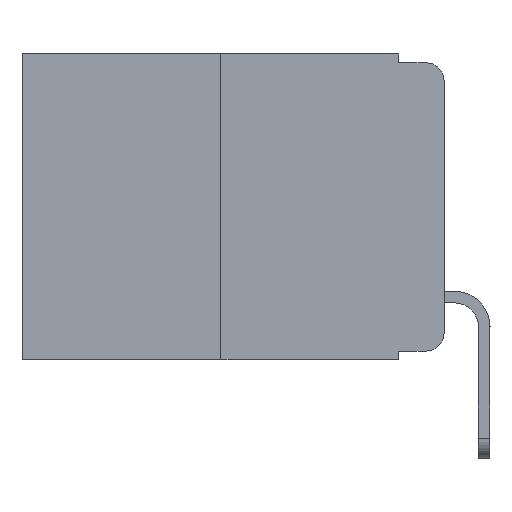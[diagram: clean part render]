
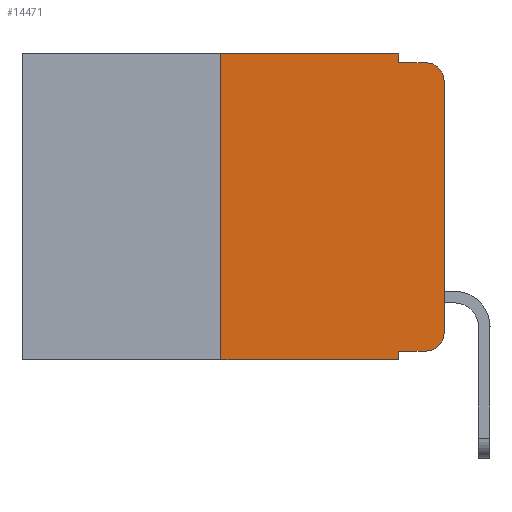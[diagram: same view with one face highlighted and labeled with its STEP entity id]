
A CAD part, left-side view. The second image highlights one B-rep face of the part: STEP entity #14471.
In plain terms, the highlighted planar face has unit normal (-1, 0, 0).
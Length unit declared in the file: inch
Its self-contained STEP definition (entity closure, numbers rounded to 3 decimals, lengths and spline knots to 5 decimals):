
#136 = EDGE_CURVE ( 'NONE', #6566, #16333, #18032, .T. ) ;
#454 = CIRCLE ( 'NONE', #20609, 0.02 ) ;
#620 = VECTOR ( 'NONE', #8441, 39.37008 ) ;
#773 = DIRECTION ( 'NONE',  ( 0., 0., -1. ) ) ;
#874 = CARTESIAN_POINT ( 'NONE',  ( 0., 0., 0. ) ) ;
#1082 = CARTESIAN_POINT ( 'NONE',  ( 0., 0.051, -0.333 ) ) ;
#1145 = ORIENTED_EDGE ( 'NONE', *, *, #17601, .F. ) ;
#1673 = AXIS2_PLACEMENT_3D ( 'NONE', #13457, #3919, #19971 ) ;
#1812 = CARTESIAN_POINT ( 'NONE',  ( 0., 0.051, -0.01 ) ) ;
#2244 = CARTESIAN_POINT ( 'NONE',  ( 0., 0.02, -0.01 ) ) ;
#2411 = DIRECTION ( 'NONE',  ( 0., -1., 0. ) ) ;
#2472 = LINE ( 'NONE', #874, #5906 ) ;
#2485 = VERTEX_POINT ( 'NONE', #20953 ) ;
#2672 = ORIENTED_EDGE ( 'NONE', *, *, #7482, .F. ) ;
#2871 = LINE ( 'NONE', #18800, #11596 ) ;
#3030 = VECTOR ( 'NONE', #3941, 39.37008 ) ;
#3312 = CARTESIAN_POINT ( 'NONE',  ( 0., 0.051, -0.01 ) ) ;
#3919 = DIRECTION ( 'NONE',  ( -1., 0., 0. ) ) ;
#3941 = DIRECTION ( 'NONE',  ( 0., -1., 0. ) ) ;
#4145 = DIRECTION ( 'NONE',  ( 0., 0., -1. ) ) ;
#4164 = LINE ( 'NONE', #1082, #3030 ) ;
#4324 = FACE_OUTER_BOUND ( 'NONE', #7030, .T. ) ;
#4434 = CARTESIAN_POINT ( 'NONE',  ( 0., 0.473, 0. ) ) ;
#4699 = CARTESIAN_POINT ( 'NONE',  ( 0., 0.25, -0.343 ) ) ;
#4918 = ORIENTED_EDGE ( 'NONE', *, *, #19283, .T. ) ;
#5364 = EDGE_CURVE ( 'NONE', #15579, #19111, #13482, .T. ) ;
#5436 = CARTESIAN_POINT ( 'NONE',  ( 0., 0.02, -0.03 ) ) ;
#5811 = ORIENTED_EDGE ( 'NONE', *, *, #136, .F. ) ;
#5906 = VECTOR ( 'NONE', #8766, 39.37008 ) ;
#5965 = EDGE_CURVE ( 'NONE', #15011, #9621, #8146, .T. ) ;
#6119 = CARTESIAN_POINT ( 'NONE',  ( 0., 0., -0.313 ) ) ;
#6271 = DIRECTION ( 'NONE',  ( 0., 0., 1. ) ) ;
#6566 = VERTEX_POINT ( 'NONE', #4699 ) ;
#6877 = LINE ( 'NONE', #18754, #10535 ) ;
#7030 = EDGE_LOOP ( 'NONE', ( #17421, #7716, #11924, #2672, #1145, #5811, #17931, #9835, #4918, #8713 ) ) ;
#7343 = CARTESIAN_POINT ( 'NONE',  ( 0., 0.473, -0.343 ) ) ;
#7482 = EDGE_CURVE ( 'NONE', #15963, #15579, #15278, .T. ) ;
#7559 = DIRECTION ( 'NONE',  ( 0., 0., -1. ) ) ;
#7569 = VERTEX_POINT ( 'NONE', #14309 ) ;
#7595 = EDGE_CURVE ( 'NONE', #6566, #8655, #15499, .T. ) ;
#7716 = ORIENTED_EDGE ( 'NONE', *, *, #12197, .T. ) ;
#7853 = PLANE ( 'NONE',  #12795 ) ;
#8031 = VECTOR ( 'NONE', #6271, 39.37008 ) ;
#8146 = CIRCLE ( 'NONE', #1673, 0.02 ) ;
#8441 = DIRECTION ( 'NONE',  ( 0., -1., 0. ) ) ;
#8655 = VERTEX_POINT ( 'NONE', #10343 ) ;
#8713 = ORIENTED_EDGE ( 'NONE', *, *, #5965, .T. ) ;
#8764 = EDGE_CURVE ( 'NONE', #7569, #8655, #2871, .T. ) ;
#8766 = DIRECTION ( 'NONE',  ( 0., 0., 1. ) ) ;
#9621 = VERTEX_POINT ( 'NONE', #6119 ) ;
#9835 = ORIENTED_EDGE ( 'NONE', *, *, #8764, .F. ) ;
#9902 = CARTESIAN_POINT ( 'NONE',  ( 0., 0.25, 0. ) ) ;
#10343 = CARTESIAN_POINT ( 'NONE',  ( 0., 0.051, -0.343 ) ) ;
#10535 = VECTOR ( 'NONE', #2411, 39.37008 ) ;
#10690 = DIRECTION ( 'NONE',  ( -1., 0., 0. ) ) ;
#10965 = DIRECTION ( 'NONE',  ( 0., 0., -1. ) ) ;
#11591 = CARTESIAN_POINT ( 'NONE',  ( 0., 0.25, 0. ) ) ;
#11596 = VECTOR ( 'NONE', #7559, 39.37008 ) ;
#11614 = VECTOR ( 'NONE', #4145, 39.37008 ) ;
#11924 = ORIENTED_EDGE ( 'NONE', *, *, #5364, .F. ) ;
#12197 = EDGE_CURVE ( 'NONE', #2485, #19111, #454, .T. ) ;
#12246 = EDGE_CURVE ( 'NONE', #9621, #2485, #2472, .T. ) ;
#12795 = AXIS2_PLACEMENT_3D ( 'NONE', #4434, #12798, #10965 ) ;
#12798 = DIRECTION ( 'NONE',  ( 1., 0., 0. ) ) ;
#13457 = CARTESIAN_POINT ( 'NONE',  ( 0., 0.02, -0.313 ) ) ;
#13482 = LINE ( 'NONE', #3312, #620 ) ;
#14001 = DIRECTION ( 'NONE',  ( 0., -1., 0. ) ) ;
#14309 = CARTESIAN_POINT ( 'NONE',  ( 0., 0.051, -0.333 ) ) ;
#14471 = ADVANCED_FACE ( 'NONE', ( #4324 ), #7853, .F. ) ;
#15011 = VERTEX_POINT ( 'NONE', #16894 ) ;
#15278 = LINE ( 'NONE', #19107, #11614 ) ;
#15499 = LINE ( 'NONE', #7343, #16344 ) ;
#15579 = VERTEX_POINT ( 'NONE', #1812 ) ;
#15963 = VERTEX_POINT ( 'NONE', #16433 ) ;
#16333 = VERTEX_POINT ( 'NONE', #11591 ) ;
#16344 = VECTOR ( 'NONE', #14001, 39.37008 ) ;
#16433 = CARTESIAN_POINT ( 'NONE',  ( 0., 0.051, 0. ) ) ;
#16894 = CARTESIAN_POINT ( 'NONE',  ( 0., 0.02, -0.333 ) ) ;
#17421 = ORIENTED_EDGE ( 'NONE', *, *, #12246, .T. ) ;
#17601 = EDGE_CURVE ( 'NONE', #16333, #15963, #6877, .T. ) ;
#17931 = ORIENTED_EDGE ( 'NONE', *, *, #7595, .T. ) ;
#18032 = LINE ( 'NONE', #9902, #8031 ) ;
#18754 = CARTESIAN_POINT ( 'NONE',  ( 0., 0.473, 0. ) ) ;
#18800 = CARTESIAN_POINT ( 'NONE',  ( 0., 0.051, 0. ) ) ;
#19107 = CARTESIAN_POINT ( 'NONE',  ( 0., 0.051, 0. ) ) ;
#19111 = VERTEX_POINT ( 'NONE', #2244 ) ;
#19283 = EDGE_CURVE ( 'NONE', #7569, #15011, #4164, .T. ) ;
#19971 = DIRECTION ( 'NONE',  ( 0., 0., -1. ) ) ;
#20609 = AXIS2_PLACEMENT_3D ( 'NONE', #5436, #10690, #773 ) ;
#20953 = CARTESIAN_POINT ( 'NONE',  ( 0., 0., -0.03 ) ) ;
